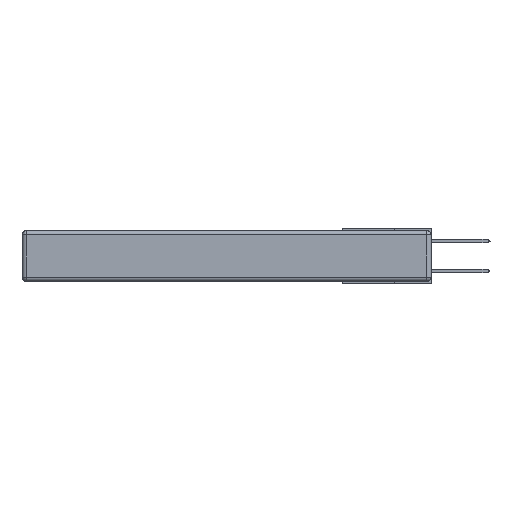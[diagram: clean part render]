
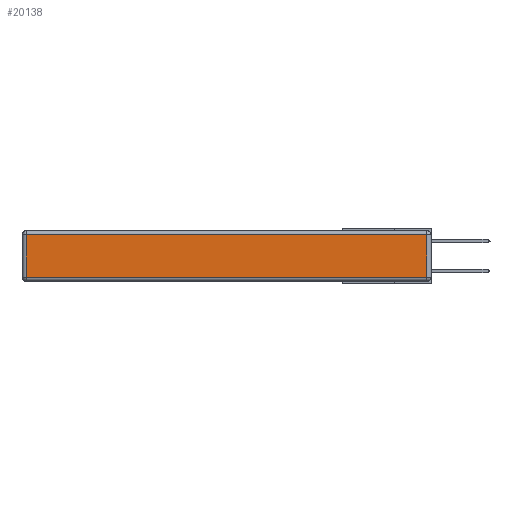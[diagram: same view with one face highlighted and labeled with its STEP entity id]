
A CAD part, left-side view. The second image highlights one B-rep face of the part: STEP entity #20138.
In plain terms, the highlighted planar face has unit normal (-1, 0, 0).
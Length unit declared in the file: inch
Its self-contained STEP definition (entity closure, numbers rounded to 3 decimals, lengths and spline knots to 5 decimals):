
#350 = VECTOR ( 'NONE', #2730, 39.37008 ) ;
#612 = VECTOR ( 'NONE', #2127, 39.37008 ) ;
#666 = AXIS2_PLACEMENT_3D ( 'NONE', #14684, #16637, #16562 ) ;
#1456 = ORIENTED_EDGE ( 'NONE', *, *, #23655, .T. ) ;
#2127 = DIRECTION ( 'NONE',  ( 0., 0., -1. ) ) ;
#2308 = ORIENTED_EDGE ( 'NONE', *, *, #13252, .T. ) ;
#2730 = DIRECTION ( 'NONE',  ( 0., 0., 1. ) ) ;
#3406 = CARTESIAN_POINT ( 'NONE',  ( 0., 0.03, -0.313 ) ) ;
#4077 = EDGE_LOOP ( 'NONE', ( #4352, #1456, #2308, #8511 ) ) ;
#4352 = ORIENTED_EDGE ( 'NONE', *, *, #19190, .T. ) ;
#6194 = LINE ( 'NONE', #10391, #10672 ) ;
#7510 = CARTESIAN_POINT ( 'NONE',  ( 0., 2.75, -0.03 ) ) ;
#8511 = ORIENTED_EDGE ( 'NONE', *, *, #11583, .T. ) ;
#9758 = VECTOR ( 'NONE', #15509, 39.37008 ) ;
#10391 = CARTESIAN_POINT ( 'NONE',  ( 0., 0., -0.313 ) ) ;
#10672 = VECTOR ( 'NONE', #23493, 39.37008 ) ;
#11108 = VERTEX_POINT ( 'NONE', #3406 ) ;
#11130 = VERTEX_POINT ( 'NONE', #20650 ) ;
#11583 = EDGE_CURVE ( 'NONE', #21224, #17443, #15408, .T. ) ;
#11821 = CARTESIAN_POINT ( 'NONE',  ( 0., 2.72, -0.343 ) ) ;
#13252 = EDGE_CURVE ( 'NONE', #11130, #21224, #20256, .T. ) ;
#13616 = CARTESIAN_POINT ( 'NONE',  ( 0., 2.72, -0.03 ) ) ;
#13645 = CARTESIAN_POINT ( 'NONE',  ( 0., 0.03, -0.343 ) ) ;
#13850 = FACE_OUTER_BOUND ( 'NONE', #4077, .T. ) ;
#14527 = PLANE ( 'NONE',  #666 ) ;
#14684 = CARTESIAN_POINT ( 'NONE',  ( 0., 0., -0.343 ) ) ;
#15408 = LINE ( 'NONE', #11821, #612 ) ;
#15509 = DIRECTION ( 'NONE',  ( 0., 1., 0. ) ) ;
#16007 = LINE ( 'NONE', #13645, #350 ) ;
#16562 = DIRECTION ( 'NONE',  ( 0., 0., 1. ) ) ;
#16637 = DIRECTION ( 'NONE',  ( -1., 0., 0. ) ) ;
#17443 = VERTEX_POINT ( 'NONE', #21018 ) ;
#19190 = EDGE_CURVE ( 'NONE', #17443, #11108, #6194, .T. ) ;
#20138 = ADVANCED_FACE ( 'NONE', ( #13850 ), #14527, .T. ) ;
#20256 = LINE ( 'NONE', #7510, #9758 ) ;
#20650 = CARTESIAN_POINT ( 'NONE',  ( 0., 0.03, -0.03 ) ) ;
#21018 = CARTESIAN_POINT ( 'NONE',  ( 0., 2.72, -0.313 ) ) ;
#21224 = VERTEX_POINT ( 'NONE', #13616 ) ;
#23493 = DIRECTION ( 'NONE',  ( 0., -1., 0. ) ) ;
#23655 = EDGE_CURVE ( 'NONE', #11108, #11130, #16007, .T. ) ;
